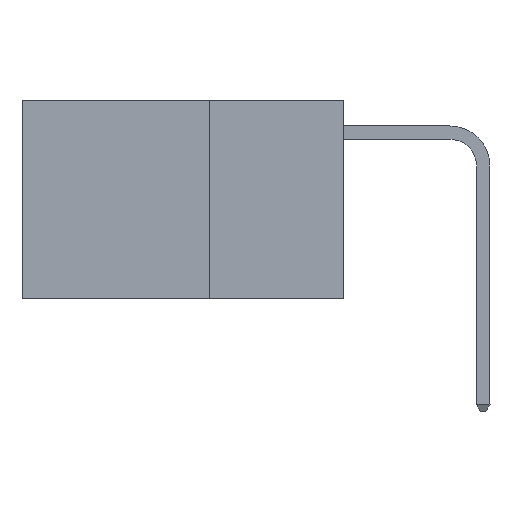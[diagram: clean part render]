
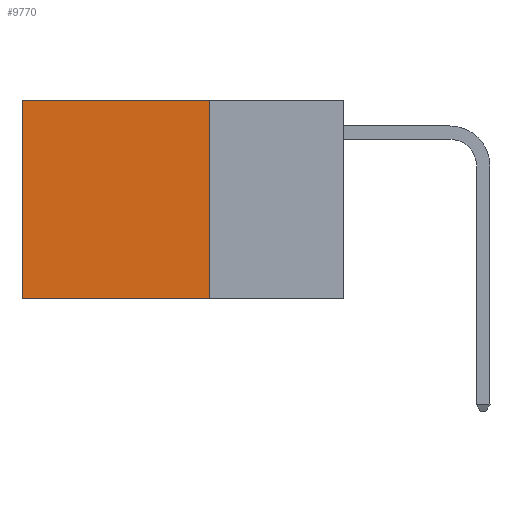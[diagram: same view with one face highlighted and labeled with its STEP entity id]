
A CAD part, left-side view. The second image highlights one B-rep face of the part: STEP entity #9770.
In plain terms, the highlighted planar face has unit normal (-1, 0, 0).
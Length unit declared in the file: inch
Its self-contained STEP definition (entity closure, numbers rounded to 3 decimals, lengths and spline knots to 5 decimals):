
#381 = LINE ( 'NONE', #8263, #12948 ) ;
#511 = EDGE_LOOP ( 'NONE', ( #6232, #2895, #14537, #7868 ) ) ;
#862 = CARTESIAN_POINT ( 'NONE',  ( 0.2625, 0.25, 0. ) ) ;
#1748 = AXIS2_PLACEMENT_3D ( 'NONE', #16192, #1881, #14925 ) ;
#1812 = EDGE_CURVE ( 'NONE', #7001, #8580, #8007, .T. ) ;
#1881 = DIRECTION ( 'NONE',  ( 1., 0., 0. ) ) ;
#2895 = ORIENTED_EDGE ( 'NONE', *, *, #4885, .F. ) ;
#3060 = DIRECTION ( 'NONE',  ( 0., 1., 0. ) ) ;
#3394 = VECTOR ( 'NONE', #6130, 39.37008 ) ;
#4468 = CARTESIAN_POINT ( 'NONE',  ( 0.2625, 0.6, -0.37 ) ) ;
#4885 = EDGE_CURVE ( 'NONE', #8580, #15511, #381, .T. ) ;
#5127 = CARTESIAN_POINT ( 'NONE',  ( 0.2625, 0.25, -0.37 ) ) ;
#5853 = FACE_OUTER_BOUND ( 'NONE', #511, .T. ) ;
#6130 = DIRECTION ( 'NONE',  ( 0., 1., 0. ) ) ;
#6232 = ORIENTED_EDGE ( 'NONE', *, *, #14003, .T. ) ;
#7001 = VERTEX_POINT ( 'NONE', #9247 ) ;
#7312 = VECTOR ( 'NONE', #10094, 39.37008 ) ;
#7405 = CARTESIAN_POINT ( 'NONE',  ( 0.2625, 0.6, 0. ) ) ;
#7868 = ORIENTED_EDGE ( 'NONE', *, *, #9414, .T. ) ;
#8007 = LINE ( 'NONE', #14615, #12746 ) ;
#8130 = PLANE ( 'NONE',  #1748 ) ;
#8263 = CARTESIAN_POINT ( 'NONE',  ( 0.2625, 0.25, -0.37 ) ) ;
#8580 = VERTEX_POINT ( 'NONE', #5127 ) ;
#8713 = VERTEX_POINT ( 'NONE', #11791 ) ;
#9247 = CARTESIAN_POINT ( 'NONE',  ( 0.2625, 0.25, 0. ) ) ;
#9414 = EDGE_CURVE ( 'NONE', #7001, #8713, #11183, .T. ) ;
#9770 = ADVANCED_FACE ( 'NONE', ( #5853 ), #8130, .F. ) ;
#10094 = DIRECTION ( 'NONE',  ( 0., 0., -1. ) ) ;
#10167 = DIRECTION ( 'NONE',  ( 0., 0., -1. ) ) ;
#11183 = LINE ( 'NONE', #862, #3394 ) ;
#11357 = LINE ( 'NONE', #7405, #7312 ) ;
#11791 = CARTESIAN_POINT ( 'NONE',  ( 0.2625, 0.6, 0. ) ) ;
#12746 = VECTOR ( 'NONE', #10167, 39.37008 ) ;
#12948 = VECTOR ( 'NONE', #3060, 39.37008 ) ;
#14003 = EDGE_CURVE ( 'NONE', #8713, #15511, #11357, .T. ) ;
#14537 = ORIENTED_EDGE ( 'NONE', *, *, #1812, .F. ) ;
#14615 = CARTESIAN_POINT ( 'NONE',  ( 0.2625, 0.25, 0. ) ) ;
#14925 = DIRECTION ( 'NONE',  ( 0., 0., -1. ) ) ;
#15511 = VERTEX_POINT ( 'NONE', #4468 ) ;
#16192 = CARTESIAN_POINT ( 'NONE',  ( 0.2625, 0.25, 0. ) ) ;
